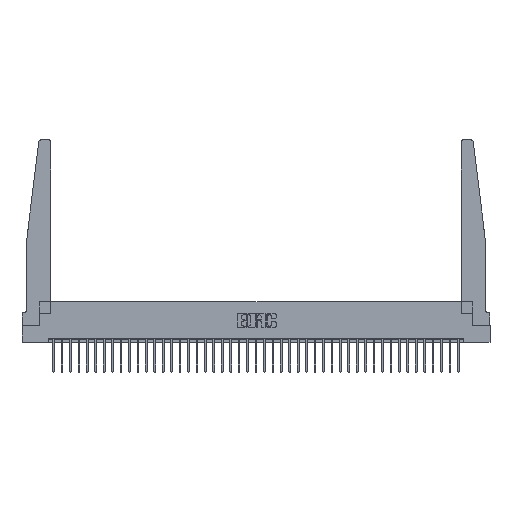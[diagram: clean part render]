
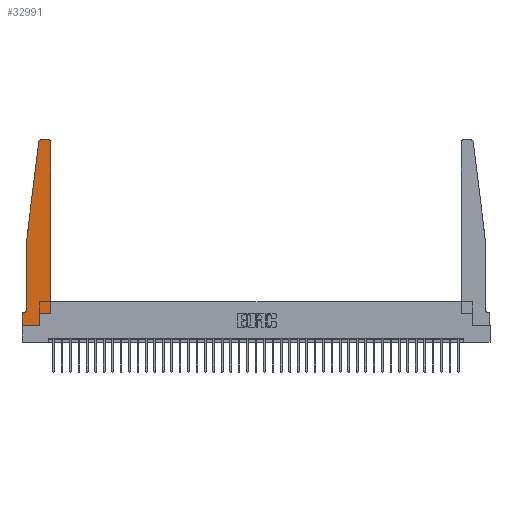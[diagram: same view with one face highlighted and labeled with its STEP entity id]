
A CAD part, top view. The second image highlights one B-rep face of the part: STEP entity #32991.
In plain terms, the highlighted planar face has unit normal (0, 0, 1).
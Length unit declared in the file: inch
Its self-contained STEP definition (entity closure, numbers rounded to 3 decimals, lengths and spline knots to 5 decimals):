
#158 = DIRECTION ( 'NONE',  ( 0., 0., 1. ) ) ;
#185 = CARTESIAN_POINT ( 'NONE',  ( 0.25, 2.75, 0.37 ) ) ;
#434 = LINE ( 'NONE', #35632, #14391 ) ;
#539 = VECTOR ( 'NONE', #24888, 39.37008 ) ;
#1320 = DIRECTION ( 'NONE',  ( -0.122, -0.992, 0. ) ) ;
#2094 = VECTOR ( 'NONE', #1320, 39.37008 ) ;
#2513 = ORIENTED_EDGE ( 'NONE', *, *, #11757, .T. ) ;
#2724 = DIRECTION ( 'NONE',  ( 0., 0., 1. ) ) ;
#3313 = EDGE_CURVE ( 'NONE', #7432, #20659, #25165, .T. ) ;
#3418 = CARTESIAN_POINT ( 'NONE',  ( 0.24675, 2.72367, 0.37 ) ) ;
#3691 = ORIENTED_EDGE ( 'NONE', *, *, #25167, .T. ) ;
#3811 = DIRECTION ( 'NONE',  ( -1., 0., 0. ) ) ;
#4548 = ORIENTED_EDGE ( 'NONE', *, *, #25190, .T. ) ;
#5003 = VERTEX_POINT ( 'NONE', #7471 ) ;
#5779 = AXIS2_PLACEMENT_3D ( 'NONE', #17131, #34200, #17196 ) ;
#6347 = CARTESIAN_POINT ( 'NONE',  ( 0.27653, 2.75, 0.37 ) ) ;
#6414 = EDGE_CURVE ( 'NONE', #27481, #10208, #23129, .T. ) ;
#6455 = CARTESIAN_POINT ( 'NONE',  ( 0.065, 0.1875, 0.37 ) ) ;
#6647 = DIRECTION ( 'NONE',  ( 0., 0., 1. ) ) ;
#7432 = VERTEX_POINT ( 'NONE', #30912 ) ;
#7471 = CARTESIAN_POINT ( 'NONE',  ( 0.425, 2.72, 0.37 ) ) ;
#7494 = DIRECTION ( 'NONE',  ( 1., 0., 0. ) ) ;
#7601 = VERTEX_POINT ( 'NONE', #3418 ) ;
#7774 = ORIENTED_EDGE ( 'NONE', *, *, #6414, .T. ) ;
#7952 = FACE_OUTER_BOUND ( 'NONE', #28629, .T. ) ;
#8595 = LINE ( 'NONE', #9684, #33310 ) ;
#9210 = CARTESIAN_POINT ( 'NONE',  ( 0.27653, 2.72, 0.37 ) ) ;
#9684 = CARTESIAN_POINT ( 'NONE',  ( 0.065, 1.25, 0.37 ) ) ;
#10000 = CARTESIAN_POINT ( 'NONE',  ( 0.2605, 0.18, 0.37 ) ) ;
#10150 = ORIENTED_EDGE ( 'NONE', *, *, #34887, .T. ) ;
#10208 = VERTEX_POINT ( 'NONE', #6347 ) ;
#10374 = CARTESIAN_POINT ( 'NONE',  ( 0.015, 0.1875, 0.37 ) ) ;
#10467 = DIRECTION ( 'NONE',  ( 0., -1., 0. ) ) ;
#10655 = LINE ( 'NONE', #21218, #20713 ) ;
#10691 = CARTESIAN_POINT ( 'NONE',  ( 0., 0., 0.37 ) ) ;
#11328 = CARTESIAN_POINT ( 'NONE',  ( 0., 0.1875, 0.37 ) ) ;
#11576 = DIRECTION ( 'NONE',  ( 1., 0., 0. ) ) ;
#11757 = EDGE_CURVE ( 'NONE', #30889, #7432, #8595, .T. ) ;
#11984 = EDGE_CURVE ( 'NONE', #28233, #5003, #17818, .T. ) ;
#12202 = EDGE_CURVE ( 'NONE', #7601, #30889, #22523, .T. ) ;
#13234 = ORIENTED_EDGE ( 'NONE', *, *, #30400, .T. ) ;
#13313 = DIRECTION ( 'NONE',  ( 1., 0., 0. ) ) ;
#13387 = CARTESIAN_POINT ( 'NONE',  ( 0.425, 0.18, 0.37 ) ) ;
#13796 = LINE ( 'NONE', #13387, #15537 ) ;
#14391 = VECTOR ( 'NONE', #13313, 39.37008 ) ;
#15444 = CARTESIAN_POINT ( 'NONE',  ( 0.065, 1.25, 0.37 ) ) ;
#15537 = VECTOR ( 'NONE', #7494, 39.37008 ) ;
#16279 = ORIENTED_EDGE ( 'NONE', *, *, #12202, .T. ) ;
#16960 = PLANE ( 'NONE',  #23152 ) ;
#17131 = CARTESIAN_POINT ( 'NONE',  ( 0.015, 0.2375, 0.37 ) ) ;
#17196 = DIRECTION ( 'NONE',  ( -1., 0., 0. ) ) ;
#17818 = LINE ( 'NONE', #35528, #25163 ) ;
#18639 = CARTESIAN_POINT ( 'NONE',  ( 0.395, 2.75, 0.37 ) ) ;
#19605 = VECTOR ( 'NONE', #10467, 39.37008 ) ;
#19934 = CARTESIAN_POINT ( 'NONE',  ( 0., 0.1875, 0.37 ) ) ;
#20468 = LINE ( 'NONE', #32860, #19605 ) ;
#20659 = VERTEX_POINT ( 'NONE', #10374 ) ;
#20713 = VECTOR ( 'NONE', #26496, 39.37008 ) ;
#20920 = DIRECTION ( 'NONE',  ( 0., -1., 0. ) ) ;
#21218 = CARTESIAN_POINT ( 'NONE',  ( 0.2605, 0.18, 0.37 ) ) ;
#22364 = CARTESIAN_POINT ( 'NONE',  ( 0.065, 1.25, 0.37 ) ) ;
#22523 = LINE ( 'NONE', #15444, #2094 ) ;
#22707 = ORIENTED_EDGE ( 'NONE', *, *, #3313, .T. ) ;
#23095 = CARTESIAN_POINT ( 'NONE',  ( 0.425, 0.18, 0.37 ) ) ;
#23105 = AXIS2_PLACEMENT_3D ( 'NONE', #9210, #6647, #25978 ) ;
#23129 = LINE ( 'NONE', #185, #539 ) ;
#23152 = AXIS2_PLACEMENT_3D ( 'NONE', #11328, #158, #11576 ) ;
#23348 = CIRCLE ( 'NONE', #23105, 0.03 ) ;
#24109 = VECTOR ( 'NONE', #3811, 39.37008 ) ;
#24477 = ORIENTED_EDGE ( 'NONE', *, *, #31986, .T. ) ;
#24821 = AXIS2_PLACEMENT_3D ( 'NONE', #33328, #2724, #30806 ) ;
#24888 = DIRECTION ( 'NONE',  ( -1., 0., 0. ) ) ;
#25163 = VECTOR ( 'NONE', #27670, 39.37008 ) ;
#25165 = CIRCLE ( 'NONE', #5779, 0.05 ) ;
#25167 = EDGE_CURVE ( 'NONE', #26029, #30220, #20468, .T. ) ;
#25190 = EDGE_CURVE ( 'NONE', #30220, #28916, #434, .T. ) ;
#25978 = DIRECTION ( 'NONE',  ( 1., 0., 0. ) ) ;
#26029 = VERTEX_POINT ( 'NONE', #19934 ) ;
#26496 = DIRECTION ( 'NONE',  ( 0., 1., 0. ) ) ;
#27481 = VERTEX_POINT ( 'NONE', #18639 ) ;
#27670 = DIRECTION ( 'NONE',  ( 0., 1., 0. ) ) ;
#27780 = ORIENTED_EDGE ( 'NONE', *, *, #11984, .T. ) ;
#28233 = VERTEX_POINT ( 'NONE', #23095 ) ;
#28629 = EDGE_LOOP ( 'NONE', ( #7774, #13234, #16279, #2513, #22707, #35656, #3691, #4548, #24477, #35590, #27780, #10150 ) ) ;
#28916 = VERTEX_POINT ( 'NONE', #32383 ) ;
#30112 = LINE ( 'NONE', #6455, #24109 ) ;
#30220 = VERTEX_POINT ( 'NONE', #10691 ) ;
#30400 = EDGE_CURVE ( 'NONE', #10208, #7601, #23348, .T. ) ;
#30639 = EDGE_CURVE ( 'NONE', #34711, #28233, #13796, .T. ) ;
#30806 = DIRECTION ( 'NONE',  ( 1., 0., 0. ) ) ;
#30889 = VERTEX_POINT ( 'NONE', #22364 ) ;
#30912 = CARTESIAN_POINT ( 'NONE',  ( 0.065, 0.2375, 0.37 ) ) ;
#31986 = EDGE_CURVE ( 'NONE', #28916, #34711, #10655, .T. ) ;
#32383 = CARTESIAN_POINT ( 'NONE',  ( 0.2605, 0., 0.37 ) ) ;
#32624 = EDGE_CURVE ( 'NONE', #20659, #26029, #30112, .T. ) ;
#32860 = CARTESIAN_POINT ( 'NONE',  ( 0., 0., 0.37 ) ) ;
#32991 = ADVANCED_FACE ( 'NONE', ( #7952 ), #16960, .T. ) ;
#33310 = VECTOR ( 'NONE', #20920, 39.37008 ) ;
#33328 = CARTESIAN_POINT ( 'NONE',  ( 0.395, 2.72, 0.37 ) ) ;
#33809 = CIRCLE ( 'NONE', #24821, 0.03 ) ;
#34200 = DIRECTION ( 'NONE',  ( 0., 0., -1. ) ) ;
#34711 = VERTEX_POINT ( 'NONE', #10000 ) ;
#34887 = EDGE_CURVE ( 'NONE', #5003, #27481, #33809, .T. ) ;
#35528 = CARTESIAN_POINT ( 'NONE',  ( 0.425, 0.18, 0.37 ) ) ;
#35590 = ORIENTED_EDGE ( 'NONE', *, *, #30639, .T. ) ;
#35632 = CARTESIAN_POINT ( 'NONE',  ( 0., 0., 0.37 ) ) ;
#35656 = ORIENTED_EDGE ( 'NONE', *, *, #32624, .T. ) ;
